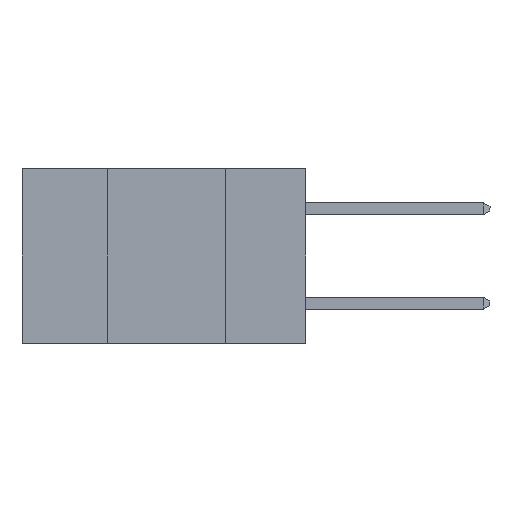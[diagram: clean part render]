
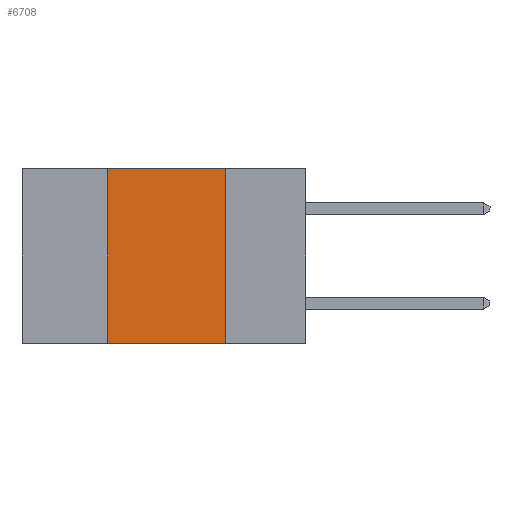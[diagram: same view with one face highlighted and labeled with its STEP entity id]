
A CAD part, left-side view. The second image highlights one B-rep face of the part: STEP entity #6708.
In plain terms, the highlighted planar face has unit normal (-1, 0, 0).
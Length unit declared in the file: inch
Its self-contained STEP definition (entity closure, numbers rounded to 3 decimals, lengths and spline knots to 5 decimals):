
#98 = ORIENTED_EDGE ( 'NONE', *, *, #9701, .F. ) ;
#294 = DIRECTION ( 'NONE',  ( 0., 0., -1. ) ) ;
#317 = VECTOR ( 'NONE', #8552, 39.37008 ) ;
#405 = EDGE_CURVE ( 'NONE', #3692, #9218, #2645, .T. ) ;
#724 = ORIENTED_EDGE ( 'NONE', *, *, #5703, .T. ) ;
#1455 = DIRECTION ( 'NONE',  ( 0., 0., 1. ) ) ;
#1510 = VECTOR ( 'NONE', #1455, 39.37008 ) ;
#1557 = LINE ( 'NONE', #3078, #5981 ) ;
#2645 = LINE ( 'NONE', #6497, #8562 ) ;
#2862 = AXIS2_PLACEMENT_3D ( 'NONE', #6346, #7095, #294 ) ;
#2928 = EDGE_LOOP ( 'NONE', ( #7498, #98, #6681, #724 ) ) ;
#3078 = CARTESIAN_POINT ( 'NONE',  ( 0., 0.6, -0.37 ) ) ;
#3692 = VERTEX_POINT ( 'NONE', #5177 ) ;
#3719 = VERTEX_POINT ( 'NONE', #5664 ) ;
#5177 = CARTESIAN_POINT ( 'NONE',  ( 0., 0.17, 0. ) ) ;
#5488 = PLANE ( 'NONE',  #2862 ) ;
#5664 = CARTESIAN_POINT ( 'NONE',  ( 0., 0.42, -0.37 ) ) ;
#5703 = EDGE_CURVE ( 'NONE', #3719, #9218, #1557, .T. ) ;
#5981 = VECTOR ( 'NONE', #7083, 39.37008 ) ;
#6134 = EDGE_CURVE ( 'NONE', #3719, #6197, #9091, .T. ) ;
#6197 = VERTEX_POINT ( 'NONE', #7783 ) ;
#6346 = CARTESIAN_POINT ( 'NONE',  ( 0., 0.6, 0. ) ) ;
#6497 = CARTESIAN_POINT ( 'NONE',  ( 0., 0.17, -0.37 ) ) ;
#6681 = ORIENTED_EDGE ( 'NONE', *, *, #6134, .F. ) ;
#6708 = ADVANCED_FACE ( 'NONE', ( #7152 ), #5488, .F. ) ;
#6946 = CARTESIAN_POINT ( 'NONE',  ( 0., 0.6, 0. ) ) ;
#7083 = DIRECTION ( 'NONE',  ( 0., -1., 0. ) ) ;
#7095 = DIRECTION ( 'NONE',  ( 1., 0., 0. ) ) ;
#7152 = FACE_OUTER_BOUND ( 'NONE', #2928, .T. ) ;
#7498 = ORIENTED_EDGE ( 'NONE', *, *, #405, .F. ) ;
#7783 = CARTESIAN_POINT ( 'NONE',  ( 0., 0.42, 0. ) ) ;
#8109 = DIRECTION ( 'NONE',  ( 0., 0., -1. ) ) ;
#8336 = CARTESIAN_POINT ( 'NONE',  ( 0., 0.42, -0.37 ) ) ;
#8552 = DIRECTION ( 'NONE',  ( 0., -1., 0. ) ) ;
#8562 = VECTOR ( 'NONE', #8109, 39.37008 ) ;
#9091 = LINE ( 'NONE', #8336, #1510 ) ;
#9218 = VERTEX_POINT ( 'NONE', #9366 ) ;
#9366 = CARTESIAN_POINT ( 'NONE',  ( 0., 0.17, -0.37 ) ) ;
#9408 = LINE ( 'NONE', #6946, #317 ) ;
#9701 = EDGE_CURVE ( 'NONE', #6197, #3692, #9408, .T. ) ;
